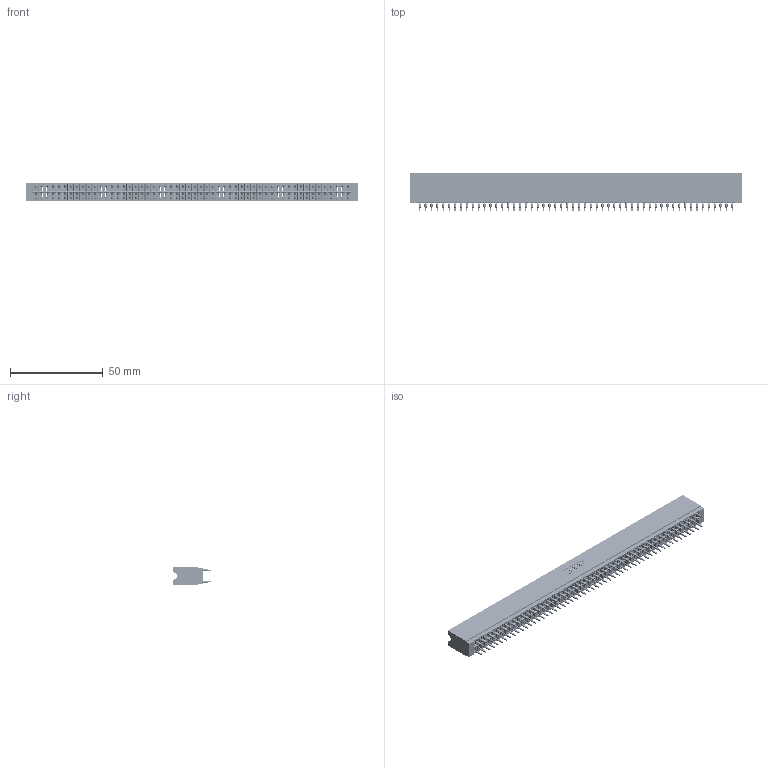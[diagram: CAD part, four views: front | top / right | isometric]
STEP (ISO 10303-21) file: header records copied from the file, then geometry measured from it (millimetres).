
FILE_DESCRIPTION (( 'STEP AP203' ), '1' );
FILE_NAME ('746-108-560-206.STEP', '2020-09-18T16:47:01', ( '' ), ( '' ), 'SwSTEP 2.0', 'SolidWorks 2020', '' );
FILE_SCHEMA (( 'CONFIG_CONTROL_DESIGN' ));
Length unit declared in the file: inch
Products named in the file (3): 746 Part_.515 Slot Depth - 06; 746-108-560-206; 746-292-001_560
Assembly tree (109 placements, depth 2):
  746-108-560-206
    746 Part_.515 Slot Depth - 06
    746-292-001_560  x108
Bounding box: 178.69 x 20.82 x 9.91 mm (x, y, z)
Volume: 19466 mm3; surface area: 33546.5 mm2
Topology: 109 solids, 109 shells, 10304 faces, 28669 edges, 18373 vertices
Faces by surface type: plane 5132, cylinder 2364, bspline 2160, torus 648
Entity records: 81850 total; most frequent: CARTESIAN_POINT 16162, ORIENTED_EDGE 14110, DIRECTION 11767, EDGE_CURVE 7055, LINE 6323, VECTOR 6323, VERTEX_POINT 4677, AXIS2_PLACEMENT_3D 2722
